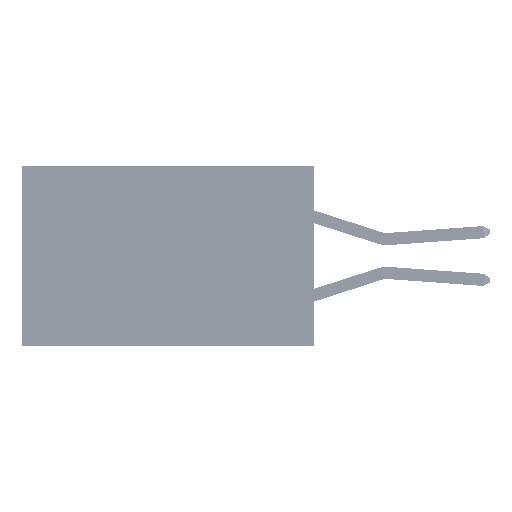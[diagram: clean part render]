
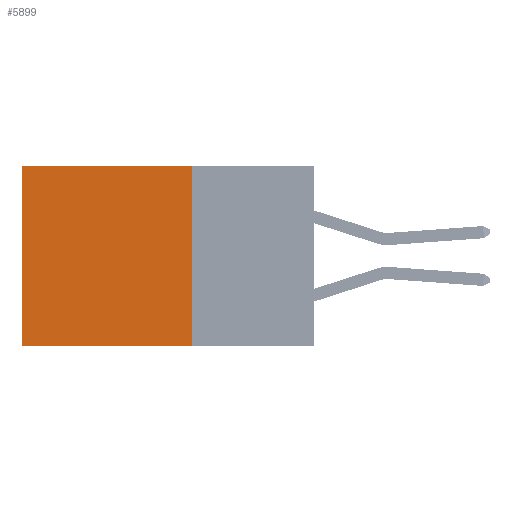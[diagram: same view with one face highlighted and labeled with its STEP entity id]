
A CAD part, left-side view. The second image highlights one B-rep face of the part: STEP entity #5899.
In plain terms, the highlighted planar face has unit normal (-1, 0, 0).
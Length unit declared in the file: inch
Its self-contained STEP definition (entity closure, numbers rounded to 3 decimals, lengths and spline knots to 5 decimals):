
#1284 = DIRECTION ( 'NONE',  ( 1., 0., 0. ) ) ;
#2142 = EDGE_CURVE ( 'NONE', #11399, #38836, #49557, .T. ) ;
#2192 = ORIENTED_EDGE ( 'NONE', *, *, #27618, .F. ) ;
#2708 = EDGE_LOOP ( 'NONE', ( #5378, #2192, #48027, #33221 ) ) ;
#2988 = LINE ( 'NONE', #21553, #32441 ) ;
#4705 = EDGE_CURVE ( 'NONE', #11399, #4771, #10463, .T. ) ;
#4771 = VERTEX_POINT ( 'NONE', #32387 ) ;
#5378 = ORIENTED_EDGE ( 'NONE', *, *, #46515, .T. ) ;
#5899 = ADVANCED_FACE ( 'NONE', ( #39708 ), #32457, .F. ) ;
#9057 = DIRECTION ( 'NONE',  ( 0., 1., 0. ) ) ;
#10463 = LINE ( 'NONE', #36916, #35523 ) ;
#11399 = VERTEX_POINT ( 'NONE', #27708 ) ;
#12806 = CARTESIAN_POINT ( 'NONE',  ( 0.2875, 0.25, 0. ) ) ;
#14287 = VERTEX_POINT ( 'NONE', #36352 ) ;
#16964 = VECTOR ( 'NONE', #17179, 39.37008 ) ;
#17179 = DIRECTION ( 'NONE',  ( 0., 0., -1. ) ) ;
#17226 = DIRECTION ( 'NONE',  ( 0., 0., -1. ) ) ;
#20559 = CARTESIAN_POINT ( 'NONE',  ( 0.2875, 0.25, 0. ) ) ;
#20666 = DIRECTION ( 'NONE',  ( 0., 1., 0. ) ) ;
#21553 = CARTESIAN_POINT ( 'NONE',  ( 0.2875, 0.6, 0. ) ) ;
#23278 = VECTOR ( 'NONE', #9057, 39.37008 ) ;
#27618 = EDGE_CURVE ( 'NONE', #38836, #14287, #35151, .T. ) ;
#27708 = CARTESIAN_POINT ( 'NONE',  ( 0.2875, 0.25, 0. ) ) ;
#29515 = CARTESIAN_POINT ( 'NONE',  ( 0.2875, 0.25, -0.37 ) ) ;
#32387 = CARTESIAN_POINT ( 'NONE',  ( 0.2875, 0.6, 0. ) ) ;
#32441 = VECTOR ( 'NONE', #46583, 39.37008 ) ;
#32457 = PLANE ( 'NONE',  #42246 ) ;
#33221 = ORIENTED_EDGE ( 'NONE', *, *, #4705, .T. ) ;
#35151 = LINE ( 'NONE', #41591, #23278 ) ;
#35523 = VECTOR ( 'NONE', #20666, 39.37008 ) ;
#36352 = CARTESIAN_POINT ( 'NONE',  ( 0.2875, 0.6, -0.37 ) ) ;
#36916 = CARTESIAN_POINT ( 'NONE',  ( 0.2875, 0.25, 0. ) ) ;
#38836 = VERTEX_POINT ( 'NONE', #29515 ) ;
#39708 = FACE_OUTER_BOUND ( 'NONE', #2708, .T. ) ;
#41591 = CARTESIAN_POINT ( 'NONE',  ( 0.2875, 0.25, -0.37 ) ) ;
#42246 = AXIS2_PLACEMENT_3D ( 'NONE', #20559, #1284, #17226 ) ;
#46515 = EDGE_CURVE ( 'NONE', #4771, #14287, #2988, .T. ) ;
#46583 = DIRECTION ( 'NONE',  ( 0., 0., -1. ) ) ;
#48027 = ORIENTED_EDGE ( 'NONE', *, *, #2142, .F. ) ;
#49557 = LINE ( 'NONE', #12806, #16964 ) ;
